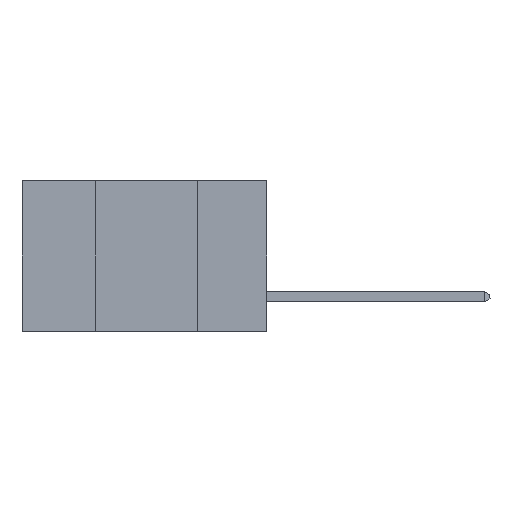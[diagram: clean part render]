
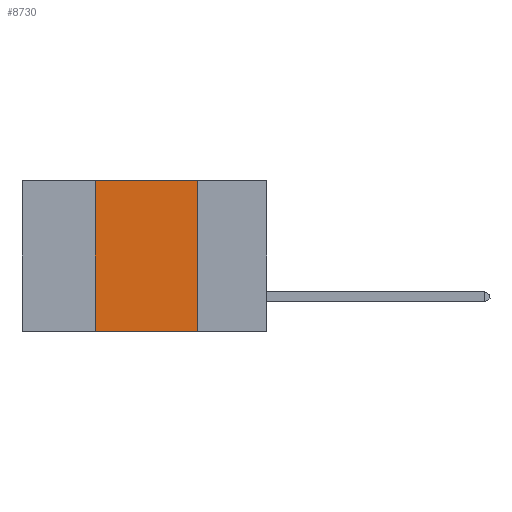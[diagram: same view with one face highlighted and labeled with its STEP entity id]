
A CAD part, left-side view. The second image highlights one B-rep face of the part: STEP entity #8730.
In plain terms, the highlighted planar face has unit normal (-1, 0, 0).
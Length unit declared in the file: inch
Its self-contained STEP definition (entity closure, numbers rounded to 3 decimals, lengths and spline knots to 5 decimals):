
#11 = DIRECTION ( 'NONE',  ( 0., 0., 1. ) ) ;
#269 = LINE ( 'NONE', #3332, #7513 ) ;
#293 = CARTESIAN_POINT ( 'NONE',  ( 0., 0.42, 0. ) ) ;
#545 = EDGE_CURVE ( 'NONE', #6693, #6209, #7157, .T. ) ;
#565 = VERTEX_POINT ( 'NONE', #580 ) ;
#580 = CARTESIAN_POINT ( 'NONE',  ( 0., 0.42, -0.37 ) ) ;
#744 = ORIENTED_EDGE ( 'NONE', *, *, #6102, .T. ) ;
#1226 = VECTOR ( 'NONE', #8072, 39.37008 ) ;
#1465 = ORIENTED_EDGE ( 'NONE', *, *, #6805, .F. ) ;
#1889 = VECTOR ( 'NONE', #3911, 39.37008 ) ;
#1965 = LINE ( 'NONE', #5801, #3684 ) ;
#2658 = DIRECTION ( 'NONE',  ( 0., -1., 0. ) ) ;
#2688 = CARTESIAN_POINT ( 'NONE',  ( 0., 0.6, 0. ) ) ;
#2845 = EDGE_LOOP ( 'NONE', ( #1465, #4942, #4154, #744 ) ) ;
#3332 = CARTESIAN_POINT ( 'NONE',  ( 0., 0.6, -0.37 ) ) ;
#3384 = DIRECTION ( 'NONE',  ( 1., 0., 0. ) ) ;
#3460 = FACE_OUTER_BOUND ( 'NONE', #2845, .T. ) ;
#3684 = VECTOR ( 'NONE', #11, 39.37008 ) ;
#3911 = DIRECTION ( 'NONE',  ( 0., -1., 0. ) ) ;
#3978 = CARTESIAN_POINT ( 'NONE',  ( 0., 0.17, -0.37 ) ) ;
#4154 = ORIENTED_EDGE ( 'NONE', *, *, #5923, .F. ) ;
#4942 = ORIENTED_EDGE ( 'NONE', *, *, #545, .F. ) ;
#5060 = LINE ( 'NONE', #7441, #1226 ) ;
#5801 = CARTESIAN_POINT ( 'NONE',  ( 0., 0.42, 0. ) ) ;
#5917 = AXIS2_PLACEMENT_3D ( 'NONE', #2688, #3384, #8027 ) ;
#5923 = EDGE_CURVE ( 'NONE', #565, #6693, #1965, .T. ) ;
#6102 = EDGE_CURVE ( 'NONE', #565, #8058, #269, .T. ) ;
#6197 = CARTESIAN_POINT ( 'NONE',  ( 0., 0.17, 0. ) ) ;
#6209 = VERTEX_POINT ( 'NONE', #6197 ) ;
#6234 = CARTESIAN_POINT ( 'NONE',  ( 0., 0.6, 0. ) ) ;
#6693 = VERTEX_POINT ( 'NONE', #293 ) ;
#6805 = EDGE_CURVE ( 'NONE', #6209, #8058, #5060, .T. ) ;
#7157 = LINE ( 'NONE', #6234, #1889 ) ;
#7399 = PLANE ( 'NONE',  #5917 ) ;
#7441 = CARTESIAN_POINT ( 'NONE',  ( 0., 0.17, 0. ) ) ;
#7513 = VECTOR ( 'NONE', #2658, 39.37008 ) ;
#8027 = DIRECTION ( 'NONE',  ( 0., 0., -1. ) ) ;
#8058 = VERTEX_POINT ( 'NONE', #3978 ) ;
#8072 = DIRECTION ( 'NONE',  ( 0., 0., -1. ) ) ;
#8730 = ADVANCED_FACE ( 'NONE', ( #3460 ), #7399, .F. ) ;
